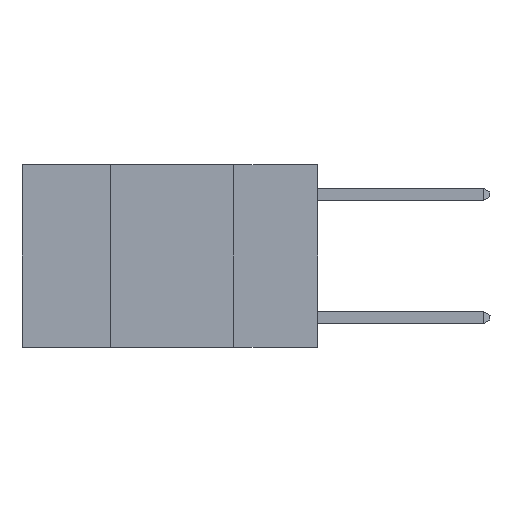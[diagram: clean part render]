
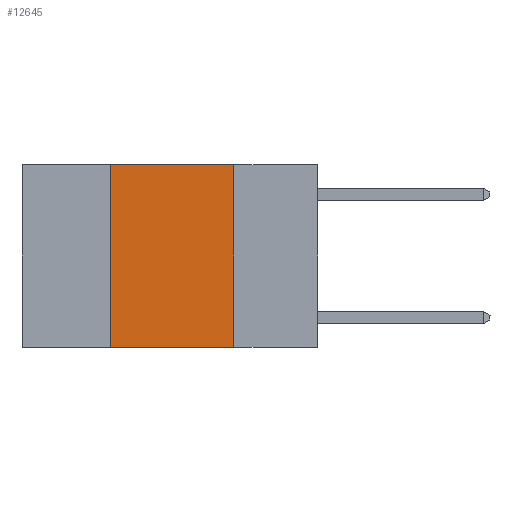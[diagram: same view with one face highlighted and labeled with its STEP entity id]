
A CAD part, left-side view. The second image highlights one B-rep face of the part: STEP entity #12645.
In plain terms, the highlighted planar face has unit normal (-1, 0, 0).
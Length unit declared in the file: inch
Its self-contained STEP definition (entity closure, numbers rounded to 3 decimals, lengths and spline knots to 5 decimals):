
#351 = CARTESIAN_POINT ( 'NONE',  ( 0., 0.42, 0. ) ) ;
#398 = EDGE_CURVE ( 'NONE', #1484, #14281, #8473, .T. ) ;
#818 = ORIENTED_EDGE ( 'NONE', *, *, #2809, .T. ) ;
#1484 = VERTEX_POINT ( 'NONE', #351 ) ;
#2437 = VECTOR ( 'NONE', #4706, 39.37008 ) ;
#2809 = EDGE_CURVE ( 'NONE', #13329, #8012, #9480, .T. ) ;
#3467 = CARTESIAN_POINT ( 'NONE',  ( 0., 0.17, -0.37 ) ) ;
#3553 = CARTESIAN_POINT ( 'NONE',  ( 0., 0.17, 0. ) ) ;
#3673 = DIRECTION ( 'NONE',  ( 0., -1., 0. ) ) ;
#4247 = ORIENTED_EDGE ( 'NONE', *, *, #398, .F. ) ;
#4253 = ORIENTED_EDGE ( 'NONE', *, *, #8729, .F. ) ;
#4295 = CARTESIAN_POINT ( 'NONE',  ( 0., 0.6, 0. ) ) ;
#4706 = DIRECTION ( 'NONE',  ( 0., 0., -1. ) ) ;
#5424 = DIRECTION ( 'NONE',  ( 0., 0., -1. ) ) ;
#5472 = VECTOR ( 'NONE', #12365, 39.37008 ) ;
#6870 = LINE ( 'NONE', #9673, #9145 ) ;
#8012 = VERTEX_POINT ( 'NONE', #3467 ) ;
#8199 = CARTESIAN_POINT ( 'NONE',  ( 0., 0.17, 0. ) ) ;
#8362 = EDGE_LOOP ( 'NONE', ( #4253, #4247, #11126, #818 ) ) ;
#8473 = LINE ( 'NONE', #12362, #5472 ) ;
#8729 = EDGE_CURVE ( 'NONE', #14281, #8012, #11123, .T. ) ;
#9145 = VECTOR ( 'NONE', #10803, 39.37008 ) ;
#9480 = LINE ( 'NONE', #11559, #12470 ) ;
#9673 = CARTESIAN_POINT ( 'NONE',  ( 0., 0.42, 0. ) ) ;
#9762 = EDGE_CURVE ( 'NONE', #13329, #1484, #6870, .T. ) ;
#9940 = FACE_OUTER_BOUND ( 'NONE', #8362, .T. ) ;
#10803 = DIRECTION ( 'NONE',  ( 0., 0., 1. ) ) ;
#11123 = LINE ( 'NONE', #3553, #2437 ) ;
#11126 = ORIENTED_EDGE ( 'NONE', *, *, #9762, .F. ) ;
#11490 = AXIS2_PLACEMENT_3D ( 'NONE', #4295, #12168, #5424 ) ;
#11559 = CARTESIAN_POINT ( 'NONE',  ( 0., 0.6, -0.37 ) ) ;
#12168 = DIRECTION ( 'NONE',  ( 1., 0., 0. ) ) ;
#12362 = CARTESIAN_POINT ( 'NONE',  ( 0., 0.6, 0. ) ) ;
#12365 = DIRECTION ( 'NONE',  ( 0., -1., 0. ) ) ;
#12470 = VECTOR ( 'NONE', #3673, 39.37008 ) ;
#12645 = ADVANCED_FACE ( 'NONE', ( #9940 ), #13229, .F. ) ;
#13229 = PLANE ( 'NONE',  #11490 ) ;
#13329 = VERTEX_POINT ( 'NONE', #14276 ) ;
#14276 = CARTESIAN_POINT ( 'NONE',  ( 0., 0.42, -0.37 ) ) ;
#14281 = VERTEX_POINT ( 'NONE', #8199 ) ;
